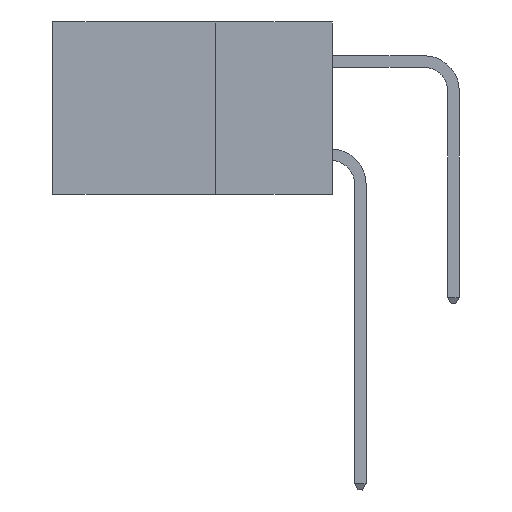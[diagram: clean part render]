
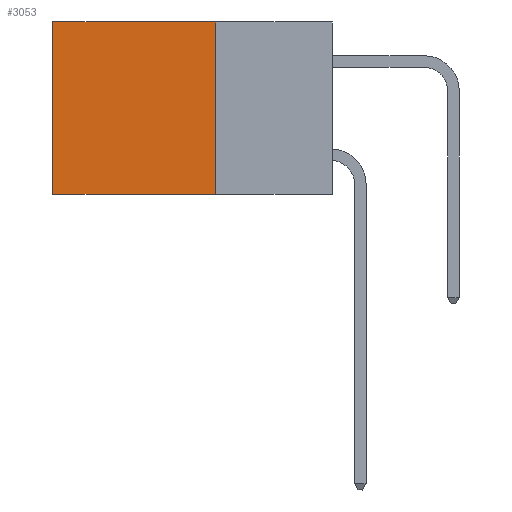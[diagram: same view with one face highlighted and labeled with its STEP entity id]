
A CAD part, left-side view. The second image highlights one B-rep face of the part: STEP entity #3053.
In plain terms, the highlighted planar face has unit normal (-1, 0, 0).
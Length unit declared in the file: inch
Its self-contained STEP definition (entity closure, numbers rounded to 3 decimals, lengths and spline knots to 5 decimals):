
#582 = CARTESIAN_POINT ( 'NONE',  ( 0.2615, 0.25, 0. ) ) ;
#767 = LINE ( 'NONE', #14323, #794 ) ;
#794 = VECTOR ( 'NONE', #14617, 39.37008 ) ;
#811 = EDGE_CURVE ( 'NONE', #14108, #1244, #10786, .T. ) ;
#1244 = VERTEX_POINT ( 'NONE', #10176 ) ;
#1860 = ORIENTED_EDGE ( 'NONE', *, *, #2305, .T. ) ;
#1955 = VERTEX_POINT ( 'NONE', #6519 ) ;
#2304 = ORIENTED_EDGE ( 'NONE', *, *, #14716, .F. ) ;
#2305 = EDGE_CURVE ( 'NONE', #5324, #14108, #9863, .T. ) ;
#2712 = CARTESIAN_POINT ( 'NONE',  ( 0.2615, 0.25, -0.37 ) ) ;
#3053 = ADVANCED_FACE ( 'NONE', ( #9219 ), #11986, .F. ) ;
#3477 = ORIENTED_EDGE ( 'NONE', *, *, #19409, .F. ) ;
#3503 = EDGE_LOOP ( 'NONE', ( #9953, #3477, #2304, #1860 ) ) ;
#5260 = VECTOR ( 'NONE', #8052, 39.37008 ) ;
#5324 = VERTEX_POINT ( 'NONE', #12373 ) ;
#6519 = CARTESIAN_POINT ( 'NONE',  ( 0.2615, 0.25, -0.37 ) ) ;
#8052 = DIRECTION ( 'NONE',  ( 0., 0., -1. ) ) ;
#8920 = DIRECTION ( 'NONE',  ( 0., 0., -1. ) ) ;
#9046 = CARTESIAN_POINT ( 'NONE',  ( 0.2615, 0.6, -0.37 ) ) ;
#9106 = CARTESIAN_POINT ( 'NONE',  ( 0.2615, 0.6, 0. ) ) ;
#9219 = FACE_OUTER_BOUND ( 'NONE', #3503, .T. ) ;
#9863 = LINE ( 'NONE', #582, #19175 ) ;
#9953 = ORIENTED_EDGE ( 'NONE', *, *, #811, .T. ) ;
#10176 = CARTESIAN_POINT ( 'NONE',  ( 0.2615, 0.6, -0.37 ) ) ;
#10786 = LINE ( 'NONE', #9046, #12938 ) ;
#11986 = PLANE ( 'NONE',  #17273 ) ;
#12373 = CARTESIAN_POINT ( 'NONE',  ( 0.2615, 0.25, 0. ) ) ;
#12418 = DIRECTION ( 'NONE',  ( 0., 0., -1. ) ) ;
#12627 = LINE ( 'NONE', #18844, #5260 ) ;
#12938 = VECTOR ( 'NONE', #12418, 39.37008 ) ;
#14108 = VERTEX_POINT ( 'NONE', #9106 ) ;
#14323 = CARTESIAN_POINT ( 'NONE',  ( 0.2615, 0.25, -0.37 ) ) ;
#14617 = DIRECTION ( 'NONE',  ( 0., 1., 0. ) ) ;
#14716 = EDGE_CURVE ( 'NONE', #5324, #1955, #12627, .T. ) ;
#16077 = DIRECTION ( 'NONE',  ( 0., 1., 0. ) ) ;
#16959 = DIRECTION ( 'NONE',  ( 1., 0., 0. ) ) ;
#17273 = AXIS2_PLACEMENT_3D ( 'NONE', #2712, #16959, #8920 ) ;
#18844 = CARTESIAN_POINT ( 'NONE',  ( 0.2615, 0.25, -0.37 ) ) ;
#19175 = VECTOR ( 'NONE', #16077, 39.37008 ) ;
#19409 = EDGE_CURVE ( 'NONE', #1955, #1244, #767, .T. ) ;
